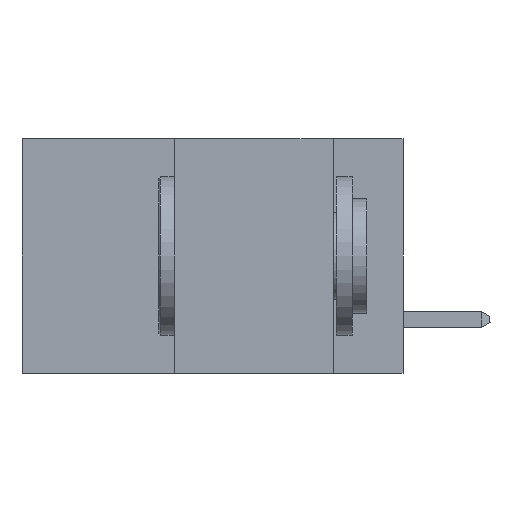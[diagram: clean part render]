
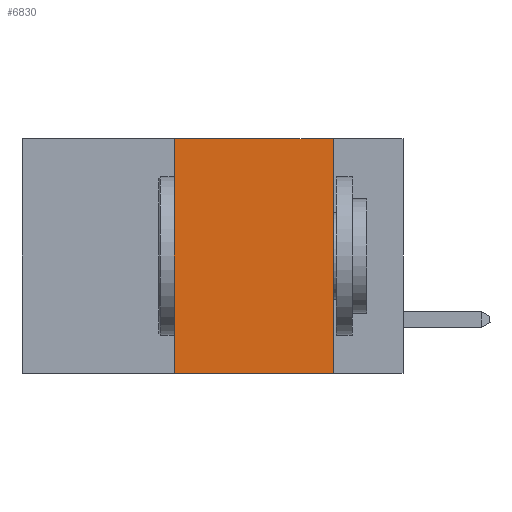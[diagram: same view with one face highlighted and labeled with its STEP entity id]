
A CAD part, left-side view. The second image highlights one B-rep face of the part: STEP entity #6830.
In plain terms, the highlighted planar face has unit normal (-1, 0, 0).
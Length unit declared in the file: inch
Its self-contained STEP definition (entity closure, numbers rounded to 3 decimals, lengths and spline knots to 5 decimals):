
#161 = CARTESIAN_POINT ( 'NONE',  ( 0., 0.11, 0. ) ) ;
#1146 = LINE ( 'NONE', #8840, #9965 ) ;
#1451 = DIRECTION ( 'NONE',  ( 0., -1., 0. ) ) ;
#1622 = EDGE_LOOP ( 'NONE', ( #8120, #1811, #10447, #9912 ) ) ;
#1811 = ORIENTED_EDGE ( 'NONE', *, *, #2135, .F. ) ;
#2135 = EDGE_CURVE ( 'NONE', #6452, #8015, #6918, .T. ) ;
#3352 = DIRECTION ( 'NONE',  ( 0., -1., 0. ) ) ;
#3759 = AXIS2_PLACEMENT_3D ( 'NONE', #5596, #5819, #11262 ) ;
#4712 = PLANE ( 'NONE',  #3759 ) ;
#5596 = CARTESIAN_POINT ( 'NONE',  ( 0., 0.6, 0. ) ) ;
#5819 = DIRECTION ( 'NONE',  ( 1., 0., 0. ) ) ;
#5988 = EDGE_CURVE ( 'NONE', #10921, #6636, #9877, .T. ) ;
#6452 = VERTEX_POINT ( 'NONE', #6891 ) ;
#6636 = VERTEX_POINT ( 'NONE', #9574 ) ;
#6830 = ADVANCED_FACE ( 'NONE', ( #8745 ), #4712, .F. ) ;
#6891 = CARTESIAN_POINT ( 'NONE',  ( 0., 0.36, 0. ) ) ;
#6918 = LINE ( 'NONE', #8413, #7320 ) ;
#7320 = VECTOR ( 'NONE', #1451, 39.37008 ) ;
#7447 = VECTOR ( 'NONE', #10712, 39.37008 ) ;
#7924 = CARTESIAN_POINT ( 'NONE',  ( 0., 0.6, -0.37 ) ) ;
#8015 = VERTEX_POINT ( 'NONE', #10629 ) ;
#8120 = ORIENTED_EDGE ( 'NONE', *, *, #10175, .F. ) ;
#8413 = CARTESIAN_POINT ( 'NONE',  ( 0., 0.6, 0. ) ) ;
#8745 = FACE_OUTER_BOUND ( 'NONE', #1622, .T. ) ;
#8840 = CARTESIAN_POINT ( 'NONE',  ( 0., 0.36, 0. ) ) ;
#9261 = LINE ( 'NONE', #161, #7447 ) ;
#9296 = EDGE_CURVE ( 'NONE', #10921, #6452, #1146, .T. ) ;
#9574 = CARTESIAN_POINT ( 'NONE',  ( 0., 0.11, -0.37 ) ) ;
#9877 = LINE ( 'NONE', #7924, #10413 ) ;
#9912 = ORIENTED_EDGE ( 'NONE', *, *, #5988, .T. ) ;
#9965 = VECTOR ( 'NONE', #10613, 39.37008 ) ;
#10175 = EDGE_CURVE ( 'NONE', #8015, #6636, #9261, .T. ) ;
#10413 = VECTOR ( 'NONE', #3352, 39.37008 ) ;
#10447 = ORIENTED_EDGE ( 'NONE', *, *, #9296, .F. ) ;
#10613 = DIRECTION ( 'NONE',  ( 0., 0., 1. ) ) ;
#10629 = CARTESIAN_POINT ( 'NONE',  ( 0., 0.11, 0. ) ) ;
#10712 = DIRECTION ( 'NONE',  ( 0., 0., -1. ) ) ;
#10859 = CARTESIAN_POINT ( 'NONE',  ( 0., 0.36, -0.37 ) ) ;
#10921 = VERTEX_POINT ( 'NONE', #10859 ) ;
#11262 = DIRECTION ( 'NONE',  ( 0., 0., -1. ) ) ;
